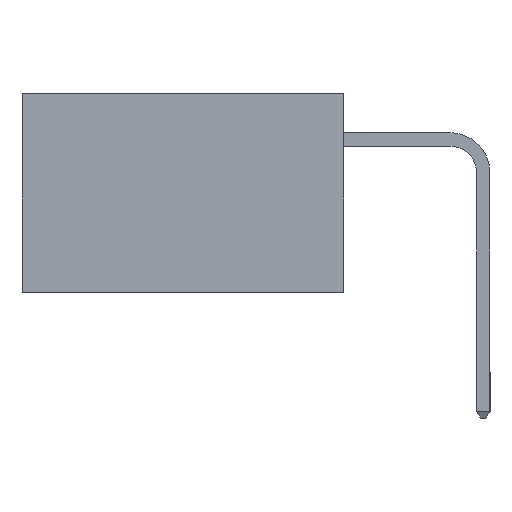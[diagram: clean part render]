
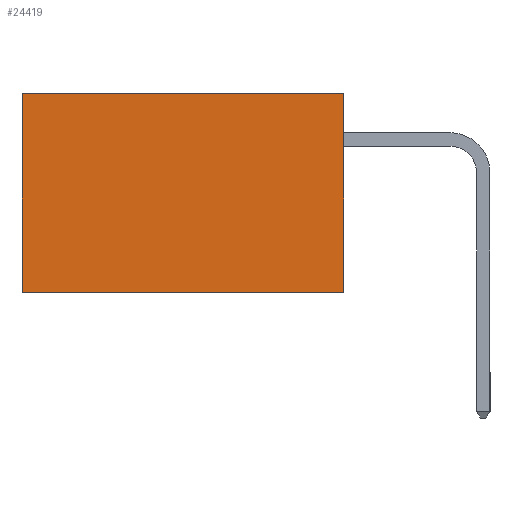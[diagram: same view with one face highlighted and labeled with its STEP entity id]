
A CAD part, left-side view. The second image highlights one B-rep face of the part: STEP entity #24419.
In plain terms, the highlighted planar face has unit normal (-1, 0, 0).
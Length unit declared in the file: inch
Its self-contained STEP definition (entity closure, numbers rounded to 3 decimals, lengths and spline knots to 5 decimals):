
#1791 = FACE_OUTER_BOUND ( 'NONE', #4416, .T. ) ;
#1971 = EDGE_CURVE ( 'NONE', #19743, #6739, #31019, .T. ) ;
#4416 = EDGE_LOOP ( 'NONE', ( #30576, #18519, #21945, #13880 ) ) ;
#5189 = VERTEX_POINT ( 'NONE', #30901 ) ;
#6739 = VERTEX_POINT ( 'NONE', #23303 ) ;
#7213 = PLANE ( 'NONE',  #30612 ) ;
#13703 = VECTOR ( 'NONE', #16694, 39.37008 ) ;
#13880 = ORIENTED_EDGE ( 'NONE', *, *, #1971, .T. ) ;
#14293 = CARTESIAN_POINT ( 'NONE',  ( 0.298, 0., -0.37 ) ) ;
#16411 = VECTOR ( 'NONE', #21517, 39.37008 ) ;
#16694 = DIRECTION ( 'NONE',  ( 0., 1., 0. ) ) ;
#17033 = DIRECTION ( 'NONE',  ( 1., 0., 0. ) ) ;
#17652 = EDGE_CURVE ( 'NONE', #23844, #5189, #26402, .T. ) ;
#17701 = EDGE_CURVE ( 'NONE', #6739, #5189, #26228, .T. ) ;
#18519 = ORIENTED_EDGE ( 'NONE', *, *, #17652, .F. ) ;
#19217 = CARTESIAN_POINT ( 'NONE',  ( 0.298, 0., 0. ) ) ;
#19596 = DIRECTION ( 'NONE',  ( 0., 0., -1. ) ) ;
#19743 = VERTEX_POINT ( 'NONE', #21910 ) ;
#20769 = DIRECTION ( 'NONE',  ( 0., 0., -1. ) ) ;
#21517 = DIRECTION ( 'NONE',  ( 0., 1., 0. ) ) ;
#21910 = CARTESIAN_POINT ( 'NONE',  ( 0.298, 0., 0. ) ) ;
#21945 = ORIENTED_EDGE ( 'NONE', *, *, #27807, .F. ) ;
#22184 = VECTOR ( 'NONE', #20769, 39.37008 ) ;
#22801 = CARTESIAN_POINT ( 'NONE',  ( 0.298, 0., 0. ) ) ;
#22946 = LINE ( 'NONE', #22801, #22184 ) ;
#23303 = CARTESIAN_POINT ( 'NONE',  ( 0.298, 0.6, 0. ) ) ;
#23844 = VERTEX_POINT ( 'NONE', #29888 ) ;
#24316 = CARTESIAN_POINT ( 'NONE',  ( 0.298, 0.6, 0. ) ) ;
#24419 = ADVANCED_FACE ( 'NONE', ( #1791 ), #7213, .F. ) ;
#26228 = LINE ( 'NONE', #24316, #30341 ) ;
#26402 = LINE ( 'NONE', #14293, #13703 ) ;
#26432 = DIRECTION ( 'NONE',  ( 0., 0., -1. ) ) ;
#27807 = EDGE_CURVE ( 'NONE', #19743, #23844, #22946, .T. ) ;
#29888 = CARTESIAN_POINT ( 'NONE',  ( 0.298, 0., -0.37 ) ) ;
#30341 = VECTOR ( 'NONE', #19596, 39.37008 ) ;
#30576 = ORIENTED_EDGE ( 'NONE', *, *, #17701, .T. ) ;
#30612 = AXIS2_PLACEMENT_3D ( 'NONE', #19217, #17033, #26432 ) ;
#30753 = CARTESIAN_POINT ( 'NONE',  ( 0.298, 0., 0. ) ) ;
#30901 = CARTESIAN_POINT ( 'NONE',  ( 0.298, 0.6, -0.37 ) ) ;
#31019 = LINE ( 'NONE', #30753, #16411 ) ;
